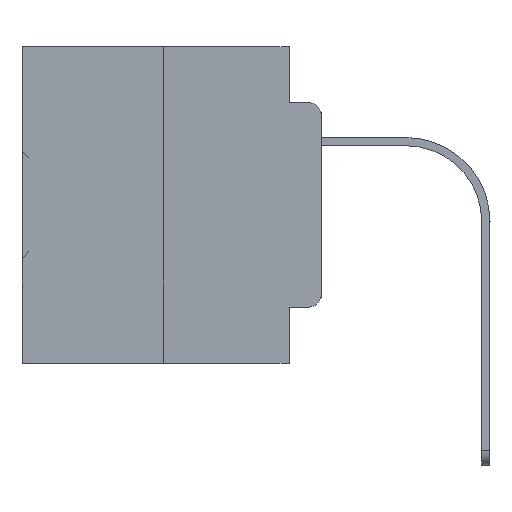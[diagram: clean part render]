
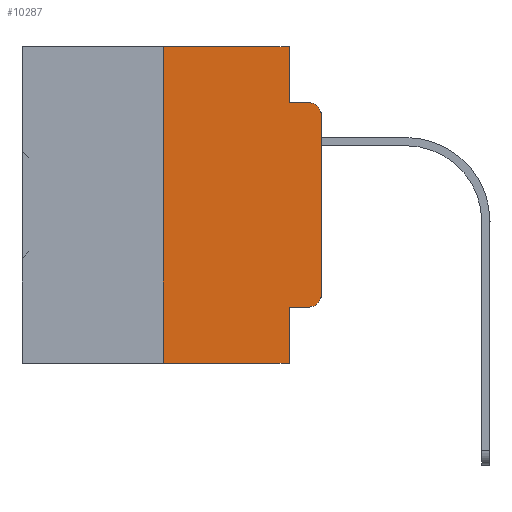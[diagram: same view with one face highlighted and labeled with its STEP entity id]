
A CAD part, left-side view. The second image highlights one B-rep face of the part: STEP entity #10287.
In plain terms, the highlighted planar face has unit normal (-1, 0, 0).
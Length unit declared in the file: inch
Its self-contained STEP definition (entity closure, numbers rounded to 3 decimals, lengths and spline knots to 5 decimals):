
#179 = CARTESIAN_POINT ( 'NONE',  ( 0., 0., -0.1085 ) ) ;
#424 = VECTOR ( 'NONE', #21069, 39.37008 ) ;
#768 = DIRECTION ( 'NONE',  ( 0., -1., 0. ) ) ;
#1533 = ORIENTED_EDGE ( 'NONE', *, *, #22130, .F. ) ;
#1730 = ORIENTED_EDGE ( 'NONE', *, *, #36692, .F. ) ;
#2011 = DIRECTION ( 'NONE',  ( 0., 0., -1. ) ) ;
#2023 = VECTOR ( 'NONE', #33392, 39.37008 ) ;
#2170 = VECTOR ( 'NONE', #22804, 39.37008 ) ;
#2238 = VECTOR ( 'NONE', #768, 39.37008 ) ;
#3015 = EDGE_CURVE ( 'NONE', #3470, #36440, #23439, .T. ) ;
#3170 = ORIENTED_EDGE ( 'NONE', *, *, #18139, .F. ) ;
#3185 = VERTEX_POINT ( 'NONE', #36902 ) ;
#3470 = VERTEX_POINT ( 'NONE', #36845 ) ;
#3578 = CARTESIAN_POINT ( 'NONE',  ( 0., 0.051, 0. ) ) ;
#5917 = DIRECTION ( 'NONE',  ( -1., 0., 0. ) ) ;
#6156 = CARTESIAN_POINT ( 'NONE',  ( 0., 0., 0. ) ) ;
#7623 = LINE ( 'NONE', #16293, #19715 ) ;
#9561 = CARTESIAN_POINT ( 'NONE',  ( 0., 0.051, -0.4115 ) ) ;
#10287 = ADVANCED_FACE ( 'NONE', ( #26672 ), #35466, .F. ) ;
#10615 = ORIENTED_EDGE ( 'NONE', *, *, #19214, .T. ) ;
#10825 = LINE ( 'NONE', #17124, #2170 ) ;
#12294 = CIRCLE ( 'NONE', #17308, 0.02 ) ;
#12562 = ORIENTED_EDGE ( 'NONE', *, *, #37943, .F. ) ;
#12710 = VERTEX_POINT ( 'NONE', #26538 ) ;
#14414 = LINE ( 'NONE', #6156, #424 ) ;
#14468 = DIRECTION ( 'NONE',  ( 0., -1., 0. ) ) ;
#14647 = CARTESIAN_POINT ( 'NONE',  ( 0., 0.051, -0.0885 ) ) ;
#15301 = DIRECTION ( 'NONE',  ( 1., 0., 0. ) ) ;
#15737 = LINE ( 'NONE', #27651, #2238 ) ;
#16251 = CARTESIAN_POINT ( 'NONE',  ( 0., 0.02, -0.4115 ) ) ;
#16293 = CARTESIAN_POINT ( 'NONE',  ( 0., 0.25, 0. ) ) ;
#16372 = VERTEX_POINT ( 'NONE', #16251 ) ;
#16715 = VECTOR ( 'NONE', #2011, 39.37008 ) ;
#17124 = CARTESIAN_POINT ( 'NONE',  ( 0., 0.473, -0.5 ) ) ;
#17308 = AXIS2_PLACEMENT_3D ( 'NONE', #19837, #34287, #31754 ) ;
#17493 = CARTESIAN_POINT ( 'NONE',  ( 0., 0.051, -0.5 ) ) ;
#18139 = EDGE_CURVE ( 'NONE', #12710, #3470, #7623, .T. ) ;
#18340 = CARTESIAN_POINT ( 'NONE',  ( 0., 0.473, 0. ) ) ;
#19214 = EDGE_CURVE ( 'NONE', #21318, #3185, #38541, .T. ) ;
#19550 = EDGE_CURVE ( 'NONE', #30987, #21318, #14414, .T. ) ;
#19715 = VECTOR ( 'NONE', #28209, 39.37008 ) ;
#19837 = CARTESIAN_POINT ( 'NONE',  ( 0., 0.02, -0.3915 ) ) ;
#21069 = DIRECTION ( 'NONE',  ( 0., 0., 1. ) ) ;
#21318 = VERTEX_POINT ( 'NONE', #179 ) ;
#21876 = VERTEX_POINT ( 'NONE', #9561 ) ;
#22130 = EDGE_CURVE ( 'NONE', #23394, #3185, #23095, .T. ) ;
#22804 = DIRECTION ( 'NONE',  ( 0., -1., 0. ) ) ;
#23095 = LINE ( 'NONE', #14647, #25018 ) ;
#23394 = VERTEX_POINT ( 'NONE', #23866 ) ;
#23439 = LINE ( 'NONE', #18340, #2023 ) ;
#23571 = CARTESIAN_POINT ( 'NONE',  ( 0., 0.02, -0.1085 ) ) ;
#23866 = CARTESIAN_POINT ( 'NONE',  ( 0., 0.051, -0.0885 ) ) ;
#24643 = EDGE_CURVE ( 'NONE', #21876, #16372, #15737, .T. ) ;
#24722 = EDGE_CURVE ( 'NONE', #16372, #30987, #12294, .T. ) ;
#25018 = VECTOR ( 'NONE', #14468, 39.37008 ) ;
#25381 = ORIENTED_EDGE ( 'NONE', *, *, #24722, .T. ) ;
#25571 = LINE ( 'NONE', #37513, #16715 ) ;
#26292 = CARTESIAN_POINT ( 'NONE',  ( 0., 0.051, 0. ) ) ;
#26538 = CARTESIAN_POINT ( 'NONE',  ( 0., 0.25, -0.5 ) ) ;
#26672 = FACE_OUTER_BOUND ( 'NONE', #34870, .T. ) ;
#27437 = ORIENTED_EDGE ( 'NONE', *, *, #19550, .T. ) ;
#27651 = CARTESIAN_POINT ( 'NONE',  ( 0., 0.051, -0.4115 ) ) ;
#28209 = DIRECTION ( 'NONE',  ( 0., 0., 1. ) ) ;
#28891 = ORIENTED_EDGE ( 'NONE', *, *, #3015, .F. ) ;
#29424 = DIRECTION ( 'NONE',  ( 0., 0., -1. ) ) ;
#29622 = EDGE_CURVE ( 'NONE', #12710, #31265, #10825, .T. ) ;
#30213 = CARTESIAN_POINT ( 'NONE',  ( 0., 0., -0.3915 ) ) ;
#30393 = VECTOR ( 'NONE', #29424, 39.37008 ) ;
#30410 = AXIS2_PLACEMENT_3D ( 'NONE', #23571, #5917, #36069 ) ;
#30987 = VERTEX_POINT ( 'NONE', #30213 ) ;
#31265 = VERTEX_POINT ( 'NONE', #17493 ) ;
#31754 = DIRECTION ( 'NONE',  ( 0., 0., -1. ) ) ;
#32547 = DIRECTION ( 'NONE',  ( 0., 0., -1. ) ) ;
#33044 = ORIENTED_EDGE ( 'NONE', *, *, #29622, .T. ) ;
#33116 = CARTESIAN_POINT ( 'NONE',  ( 0., 0.473, 0. ) ) ;
#33392 = DIRECTION ( 'NONE',  ( 0., -1., 0. ) ) ;
#34287 = DIRECTION ( 'NONE',  ( -1., 0., 0. ) ) ;
#34870 = EDGE_LOOP ( 'NONE', ( #27437, #10615, #1533, #1730, #28891, #3170, #33044, #12562, #38127, #25381 ) ) ;
#35466 = PLANE ( 'NONE',  #38265 ) ;
#36057 = LINE ( 'NONE', #26292, #30393 ) ;
#36069 = DIRECTION ( 'NONE',  ( 0., 0., -1. ) ) ;
#36440 = VERTEX_POINT ( 'NONE', #3578 ) ;
#36692 = EDGE_CURVE ( 'NONE', #36440, #23394, #36057, .T. ) ;
#36845 = CARTESIAN_POINT ( 'NONE',  ( 0., 0.25, 0. ) ) ;
#36902 = CARTESIAN_POINT ( 'NONE',  ( 0., 0.02, -0.0885 ) ) ;
#37513 = CARTESIAN_POINT ( 'NONE',  ( 0., 0.051, 0. ) ) ;
#37943 = EDGE_CURVE ( 'NONE', #21876, #31265, #25571, .T. ) ;
#38127 = ORIENTED_EDGE ( 'NONE', *, *, #24643, .T. ) ;
#38265 = AXIS2_PLACEMENT_3D ( 'NONE', #33116, #15301, #32547 ) ;
#38541 = CIRCLE ( 'NONE', #30410, 0.02 ) ;
